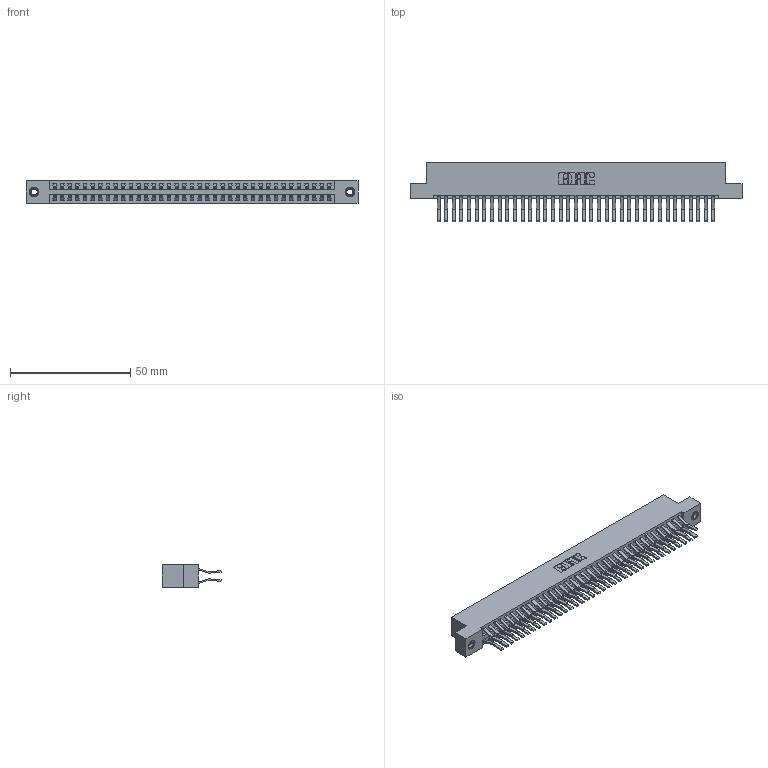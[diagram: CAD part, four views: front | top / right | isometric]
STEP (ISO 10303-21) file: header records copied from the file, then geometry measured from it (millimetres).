
FILE_DESCRIPTION (( 'STEP AP203' ), '1' );
FILE_NAME ('396-074-560-207.STEP', '2019-10-30T21:02:30', ( '' ), ( '' ), 'SwSTEP 2.0', 'SolidWorks 2016', '' );
FILE_SCHEMA (( 'CONFIG_CONTROL_DESIGN' ));
Length unit declared in the file: inch
Products named in the file (4): 345-292-001_560 Tail; 396-074-560-207; 345-250-001_345-250-005-103; 346 Part_Flush Mounting Lugs - 0.156 Dia-TI
Assembly tree (77 placements, depth 2):
  396-074-560-207
    346 Part_Flush Mounting Lugs - 0.156 Dia-TI
    345-292-001_560 Tail  x74
    345-250-001_345-250-005-103  x2
Bounding box: 138.05 x 24.78 x 9.4 mm (x, y, z)
Volume: 13894.2 mm3; surface area: 20347.7 mm2
Topology: 77 solids, 77 shells, 4178 faces, 12379 edges, 8146 vertices
Faces by surface type: plane 2698, cylinder 1464, cone 12, torus 4
Entity records: 26094 total; most frequent: CARTESIAN_POINT 4291, ORIENTED_EDGE 4218, DIRECTION 3863, EDGE_CURVE 2109, LINE 1805, VECTOR 1805, VERTEX_POINT 1400, AXIS2_PLACEMENT_3D 1029
